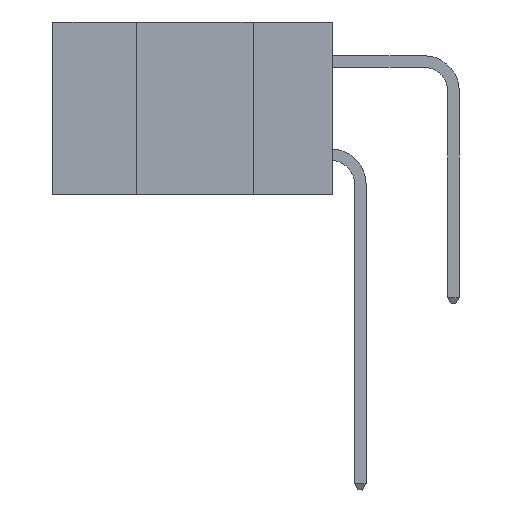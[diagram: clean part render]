
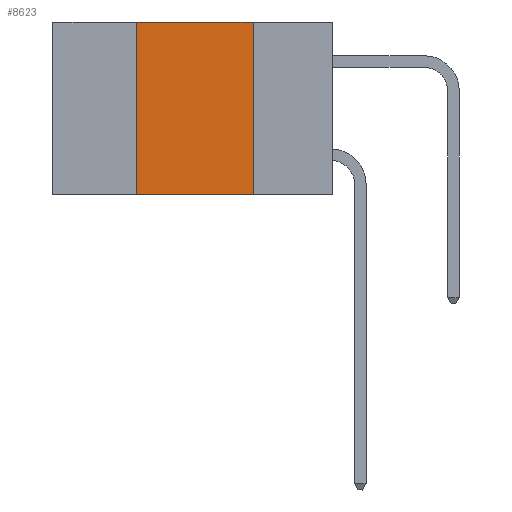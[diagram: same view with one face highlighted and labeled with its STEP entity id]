
A CAD part, left-side view. The second image highlights one B-rep face of the part: STEP entity #8623.
In plain terms, the highlighted planar face has unit normal (-1, 0, 0).
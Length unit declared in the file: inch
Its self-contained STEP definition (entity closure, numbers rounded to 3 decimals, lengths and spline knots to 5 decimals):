
#112 = DIRECTION ( 'NONE',  ( 0., 0., 1. ) ) ;
#207 = ORIENTED_EDGE ( 'NONE', *, *, #7903, .F. ) ;
#560 = DIRECTION ( 'NONE',  ( 0., -1., 0. ) ) ;
#569 = VERTEX_POINT ( 'NONE', #17306 ) ;
#1127 = VERTEX_POINT ( 'NONE', #9441 ) ;
#1933 = ORIENTED_EDGE ( 'NONE', *, *, #15218, .T. ) ;
#2886 = CARTESIAN_POINT ( 'NONE',  ( 0., 0.6, 0. ) ) ;
#3788 = CARTESIAN_POINT ( 'NONE',  ( 0., 0.6, -0.37 ) ) ;
#3833 = DIRECTION ( 'NONE',  ( 0., -1., 0. ) ) ;
#3993 = LINE ( 'NONE', #16413, #10566 ) ;
#4455 = DIRECTION ( 'NONE',  ( 1., 0., 0. ) ) ;
#5560 = EDGE_CURVE ( 'NONE', #1127, #9943, #17016, .T. ) ;
#6514 = VECTOR ( 'NONE', #3833, 39.37008 ) ;
#7061 = DIRECTION ( 'NONE',  ( 0., 0., -1. ) ) ;
#7482 = EDGE_CURVE ( 'NONE', #15801, #1127, #18399, .T. ) ;
#7903 = EDGE_CURVE ( 'NONE', #9943, #569, #3993, .T. ) ;
#8253 = CARTESIAN_POINT ( 'NONE',  ( 0., 0.42, -0.37 ) ) ;
#8384 = CARTESIAN_POINT ( 'NONE',  ( 0., 0.6, 0. ) ) ;
#8623 = ADVANCED_FACE ( 'NONE', ( #10790 ), #18155, .F. ) ;
#8675 = ORIENTED_EDGE ( 'NONE', *, *, #7482, .F. ) ;
#9019 = EDGE_LOOP ( 'NONE', ( #207, #18128, #8675, #1933 ) ) ;
#9441 = CARTESIAN_POINT ( 'NONE',  ( 0., 0.42, 0. ) ) ;
#9943 = VERTEX_POINT ( 'NONE', #18766 ) ;
#10566 = VECTOR ( 'NONE', #7061, 39.37008 ) ;
#10790 = FACE_OUTER_BOUND ( 'NONE', #9019, .T. ) ;
#12721 = CARTESIAN_POINT ( 'NONE',  ( 0., 0.42, 0. ) ) ;
#15218 = EDGE_CURVE ( 'NONE', #15801, #569, #18811, .T. ) ;
#15801 = VERTEX_POINT ( 'NONE', #8253 ) ;
#16413 = CARTESIAN_POINT ( 'NONE',  ( 0., 0.17, 0. ) ) ;
#16954 = DIRECTION ( 'NONE',  ( 0., 0., -1. ) ) ;
#17016 = LINE ( 'NONE', #8384, #6514 ) ;
#17306 = CARTESIAN_POINT ( 'NONE',  ( 0., 0.17, -0.37 ) ) ;
#18128 = ORIENTED_EDGE ( 'NONE', *, *, #5560, .F. ) ;
#18155 = PLANE ( 'NONE',  #19883 ) ;
#18324 = VECTOR ( 'NONE', #560, 39.37008 ) ;
#18399 = LINE ( 'NONE', #12721, #18633 ) ;
#18633 = VECTOR ( 'NONE', #112, 39.37008 ) ;
#18766 = CARTESIAN_POINT ( 'NONE',  ( 0., 0.17, 0. ) ) ;
#18811 = LINE ( 'NONE', #3788, #18324 ) ;
#19883 = AXIS2_PLACEMENT_3D ( 'NONE', #2886, #4455, #16954 ) ;
